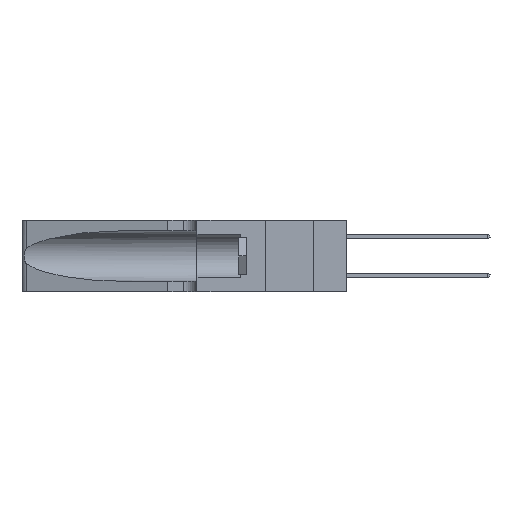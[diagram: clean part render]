
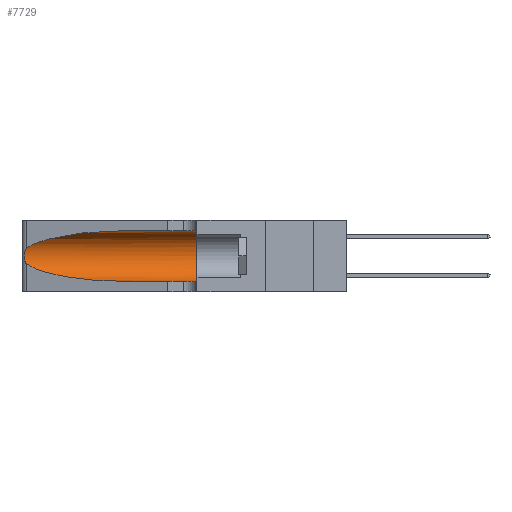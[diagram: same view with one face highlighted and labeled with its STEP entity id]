
A CAD part, left-side view. The second image highlights one B-rep face of the part: STEP entity #7729.
In plain terms, the highlighted cylindrical face has radius 3.308 mm (diameter 6.617 mm), a partial arc.
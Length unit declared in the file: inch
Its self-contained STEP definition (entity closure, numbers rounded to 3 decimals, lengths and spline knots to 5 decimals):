
#166 =( BOUNDED_CURVE ( )  B_SPLINE_CURVE ( 3, ( #34161, #9163, #16512, #41256 ),
 .UNSPECIFIED., .F., .F. ) 
 B_SPLINE_CURVE_WITH_KNOTS ( ( 4, 4 ),
 ( 3.44316, 4.71239 ),
 .UNSPECIFIED. ) 
 CURVE ( )  GEOMETRIC_REPRESENTATION_ITEM ( )  RATIONAL_B_SPLINE_CURVE ( ( 1., 0.87, 0.87, 1. ) ) 
 REPRESENTATION_ITEM ( '' )  );
#1757 = CARTESIAN_POINT ( 'NONE',  ( 0.1305, 1.61858, 0.05475 ) ) ;
#3454 = CARTESIAN_POINT ( 'NONE',  ( 0.26017, 1.23833, 0.17102 ) ) ;
#5337 = CARTESIAN_POINT ( 'NONE',  ( 0.2373, 1.15595, 0.28018 ) ) ;
#6274 = VECTOR ( 'NONE', #14238, 39.37008 ) ;
#7105 = CARTESIAN_POINT ( 'NONE',  ( 0.25789, 1.23486, 0.15765 ) ) ;
#7647 = VERTEX_POINT ( 'NONE', #34180 ) ;
#7702 = DIRECTION ( 'NONE',  ( 0., 1., 0. ) ) ;
#7729 = ADVANCED_FACE ( 'NONE', ( #44414 ), #24502, .F. ) ;
#7787 = EDGE_CURVE ( 'NONE', #11322, #27904, #8621, .T. ) ;
#8621 = B_SPLINE_CURVE_WITH_KNOTS ( 'NONE', 3,
 ( #13698, #34938, #9976, #17323, #42054, #20901, #45641, #24482, #3454, #28648, #7105, #32194, #10768, #35719 ),
 .UNSPECIFIED., .F., .F.,
 ( 4, 2, 2, 2, 2, 2, 4 ),
 ( 0., 0.00027, 0.00053, 0.00107, 0.0016, 0.00187, 0.00214 ),
 .UNSPECIFIED. ) ;
#9163 = CARTESIAN_POINT ( 'NONE',  ( 0.2373, 1.15595, 0.08982 ) ) ;
#9329 = CARTESIAN_POINT ( 'NONE',  ( 0.1305, 0.72297, 0.05475 ) ) ;
#9656 = DIRECTION ( 'NONE',  ( 0., 0., -1. ) ) ;
#9976 = CARTESIAN_POINT ( 'NONE',  ( 0.25639, 1.23184, 0.21858 ) ) ;
#10768 = CARTESIAN_POINT ( 'NONE',  ( 0.25555, 1.22993, 0.14849 ) ) ;
#11322 = VERTEX_POINT ( 'NONE', #22205 ) ;
#11598 = EDGE_CURVE ( 'NONE', #16305, #32525, #26459, .T. ) ;
#12928 = DIRECTION ( 'NONE',  ( 0., -1., 0. ) ) ;
#13639 = ORIENTED_EDGE ( 'NONE', *, *, #11598, .T. ) ;
#13648 = AXIS2_PLACEMENT_3D ( 'NONE', #29243, #7702, #32777 ) ;
#13698 = CARTESIAN_POINT ( 'NONE',  ( 0.25487, 1.22718, 0.22369 ) ) ;
#14238 = DIRECTION ( 'NONE',  ( 0., -1., 0. ) ) ;
#14344 = EDGE_LOOP ( 'NONE', ( #21437, #44721, #40786, #13639, #41910, #28685 ) ) ;
#15086 = EDGE_CURVE ( 'NONE', #27904, #16305, #166, .T. ) ;
#16305 = VERTEX_POINT ( 'NONE', #9329 ) ;
#16512 = CARTESIAN_POINT ( 'NONE',  ( 0.18966, 0.96281, 0.05475 ) ) ;
#17183 = EDGE_CURVE ( 'NONE', #7647, #42231, #42006, .T. ) ;
#17323 = CARTESIAN_POINT ( 'NONE',  ( 0.25787, 1.23484, 0.2124 ) ) ;
#17702 = CARTESIAN_POINT ( 'NONE',  ( 0.1305, 1.61858, 0.31525 ) ) ;
#20901 = CARTESIAN_POINT ( 'NONE',  ( 0.26018, 1.23835, 0.19895 ) ) ;
#20919 = EDGE_CURVE ( 'NONE', #7647, #11322, #38389, .T. ) ;
#21437 = ORIENTED_EDGE ( 'NONE', *, *, #20919, .T. ) ;
#22205 = CARTESIAN_POINT ( 'NONE',  ( 0.25487, 1.22718, 0.22369 ) ) ;
#23361 = CARTESIAN_POINT ( 'NONE',  ( 0.1305, 0.72297, 0.31525 ) ) ;
#24482 = CARTESIAN_POINT ( 'NONE',  ( 0.26075, 1.23896, 0.178 ) ) ;
#24502 = CYLINDRICAL_SURFACE ( 'NONE', #40216, 0.13025 ) ;
#26459 = LINE ( 'NONE', #1757, #44116 ) ;
#26934 = CARTESIAN_POINT ( 'NONE',  ( 0.25487, 1.22718, 0.14631 ) ) ;
#27904 = VERTEX_POINT ( 'NONE', #26934 ) ;
#28648 = CARTESIAN_POINT ( 'NONE',  ( 0.25856, 1.23593, 0.16098 ) ) ;
#28685 = ORIENTED_EDGE ( 'NONE', *, *, #17183, .F. ) ;
#29243 = CARTESIAN_POINT ( 'NONE',  ( 0.1305, 0.35, 0.185 ) ) ;
#30471 = CARTESIAN_POINT ( 'NONE',  ( 0.25487, 1.22718, 0.22369 ) ) ;
#32194 = CARTESIAN_POINT ( 'NONE',  ( 0.25639, 1.23186, 0.15144 ) ) ;
#32525 = VERTEX_POINT ( 'NONE', #39253 ) ;
#32777 = DIRECTION ( 'NONE',  ( 0., 0., 1. ) ) ;
#34161 = CARTESIAN_POINT ( 'NONE',  ( 0.25487, 1.22718, 0.14631 ) ) ;
#34180 = CARTESIAN_POINT ( 'NONE',  ( 0.1305, 0.72297, 0.31525 ) ) ;
#34647 = DIRECTION ( 'NONE',  ( 0., -1., 0. ) ) ;
#34938 = CARTESIAN_POINT ( 'NONE',  ( 0.25555, 1.22994, 0.2215 ) ) ;
#35719 = CARTESIAN_POINT ( 'NONE',  ( 0.25487, 1.22718, 0.14631 ) ) ;
#36677 = CIRCLE ( 'NONE', #13648, 0.13025 ) ;
#38389 =( BOUNDED_CURVE ( )  B_SPLINE_CURVE ( 3, ( #23361, #44543, #5337, #30471 ),
 .UNSPECIFIED., .F., .F. ) 
 B_SPLINE_CURVE_WITH_KNOTS ( ( 4, 4 ),
 ( 1.5708, 2.84003 ),
 .UNSPECIFIED. ) 
 CURVE ( )  GEOMETRIC_REPRESENTATION_ITEM ( )  RATIONAL_B_SPLINE_CURVE ( ( 1., 0.87, 0.87, 1. ) ) 
 REPRESENTATION_ITEM ( '' )  );
#39253 = CARTESIAN_POINT ( 'NONE',  ( 0.1305, 0.35, 0.05475 ) ) ;
#40216 = AXIS2_PLACEMENT_3D ( 'NONE', #41747, #34647, #9656 ) ;
#40786 = ORIENTED_EDGE ( 'NONE', *, *, #15086, .T. ) ;
#41256 = CARTESIAN_POINT ( 'NONE',  ( 0.1305, 0.72297, 0.05475 ) ) ;
#41747 = CARTESIAN_POINT ( 'NONE',  ( 0.1305, 1.61858, 0.185 ) ) ;
#41910 = ORIENTED_EDGE ( 'NONE', *, *, #45219, .F. ) ;
#42006 = LINE ( 'NONE', #17702, #6274 ) ;
#42054 = CARTESIAN_POINT ( 'NONE',  ( 0.25854, 1.2359, 0.20912 ) ) ;
#42231 = VERTEX_POINT ( 'NONE', #44602 ) ;
#44116 = VECTOR ( 'NONE', #12928, 39.37008 ) ;
#44414 = FACE_OUTER_BOUND ( 'NONE', #14344, .T. ) ;
#44543 = CARTESIAN_POINT ( 'NONE',  ( 0.18966, 0.96281, 0.31525 ) ) ;
#44602 = CARTESIAN_POINT ( 'NONE',  ( 0.1305, 0.35, 0.31525 ) ) ;
#44721 = ORIENTED_EDGE ( 'NONE', *, *, #7787, .T. ) ;
#45219 = EDGE_CURVE ( 'NONE', #42231, #32525, #36677, .T. ) ;
#45641 = CARTESIAN_POINT ( 'NONE',  ( 0.26075, 1.23896, 0.19203 ) ) ;
